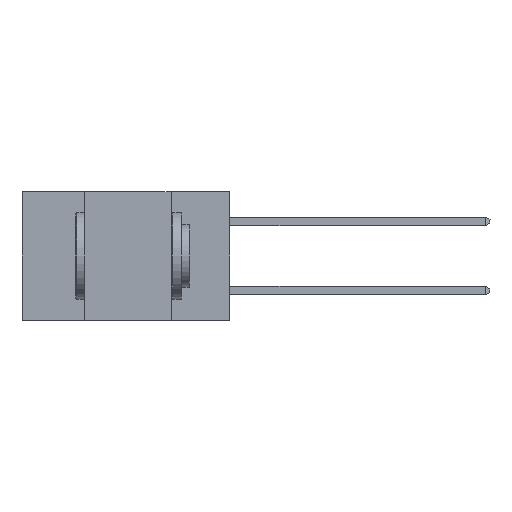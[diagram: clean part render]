
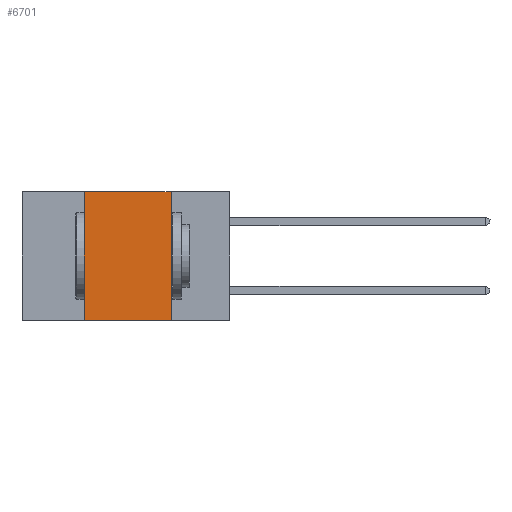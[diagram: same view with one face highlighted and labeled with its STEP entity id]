
A CAD part, left-side view. The second image highlights one B-rep face of the part: STEP entity #6701.
In plain terms, the highlighted planar face has unit normal (-1, 0, 0).
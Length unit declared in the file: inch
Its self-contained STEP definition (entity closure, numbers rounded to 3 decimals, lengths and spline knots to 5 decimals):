
#158 = EDGE_CURVE ( 'NONE', #1566, #8327, #1307, .T. ) ;
#230 = CARTESIAN_POINT ( 'NONE',  ( 0., 0.17, 0. ) ) ;
#292 = VECTOR ( 'NONE', #8767, 39.37008 ) ;
#1014 = ORIENTED_EDGE ( 'NONE', *, *, #3522, .T. ) ;
#1307 = LINE ( 'NONE', #1982, #292 ) ;
#1566 = VERTEX_POINT ( 'NONE', #8708 ) ;
#1711 = VECTOR ( 'NONE', #5955, 39.37008 ) ;
#1982 = CARTESIAN_POINT ( 'NONE',  ( 0., 0.42, -0.37 ) ) ;
#1992 = LINE ( 'NONE', #6539, #4734 ) ;
#2275 = DIRECTION ( 'NONE',  ( 1., 0., 0. ) ) ;
#2342 = CARTESIAN_POINT ( 'NONE',  ( 0., 0.17, -0.37 ) ) ;
#3063 = LINE ( 'NONE', #2342, #5627 ) ;
#3251 = CARTESIAN_POINT ( 'NONE',  ( 0., 0.17, -0.37 ) ) ;
#3450 = ORIENTED_EDGE ( 'NONE', *, *, #4870, .F. ) ;
#3493 = EDGE_LOOP ( 'NONE', ( #3450, #6214, #8499, #1014 ) ) ;
#3522 = EDGE_CURVE ( 'NONE', #1566, #3687, #8157, .T. ) ;
#3687 = VERTEX_POINT ( 'NONE', #3251 ) ;
#4035 = VERTEX_POINT ( 'NONE', #230 ) ;
#4420 = DIRECTION ( 'NONE',  ( 0., 0., -1. ) ) ;
#4734 = VECTOR ( 'NONE', #8100, 39.37008 ) ;
#4870 = EDGE_CURVE ( 'NONE', #4035, #3687, #3063, .T. ) ;
#5627 = VECTOR ( 'NONE', #8248, 39.37008 ) ;
#5940 = CARTESIAN_POINT ( 'NONE',  ( 0., 0.6, 0. ) ) ;
#5955 = DIRECTION ( 'NONE',  ( 0., -1., 0. ) ) ;
#6214 = ORIENTED_EDGE ( 'NONE', *, *, #7857, .F. ) ;
#6539 = CARTESIAN_POINT ( 'NONE',  ( 0., 0.6, 0. ) ) ;
#6701 = ADVANCED_FACE ( 'NONE', ( #6726 ), #9067, .F. ) ;
#6726 = FACE_OUTER_BOUND ( 'NONE', #3493, .T. ) ;
#7376 = CARTESIAN_POINT ( 'NONE',  ( 0., 0.6, -0.37 ) ) ;
#7542 = CARTESIAN_POINT ( 'NONE',  ( 0., 0.42, 0. ) ) ;
#7857 = EDGE_CURVE ( 'NONE', #8327, #4035, #1992, .T. ) ;
#8100 = DIRECTION ( 'NONE',  ( 0., -1., 0. ) ) ;
#8157 = LINE ( 'NONE', #7376, #1711 ) ;
#8248 = DIRECTION ( 'NONE',  ( 0., 0., -1. ) ) ;
#8327 = VERTEX_POINT ( 'NONE', #7542 ) ;
#8499 = ORIENTED_EDGE ( 'NONE', *, *, #158, .F. ) ;
#8708 = CARTESIAN_POINT ( 'NONE',  ( 0., 0.42, -0.37 ) ) ;
#8767 = DIRECTION ( 'NONE',  ( 0., 0., 1. ) ) ;
#9067 = PLANE ( 'NONE',  #9259 ) ;
#9259 = AXIS2_PLACEMENT_3D ( 'NONE', #5940, #2275, #4420 ) ;
